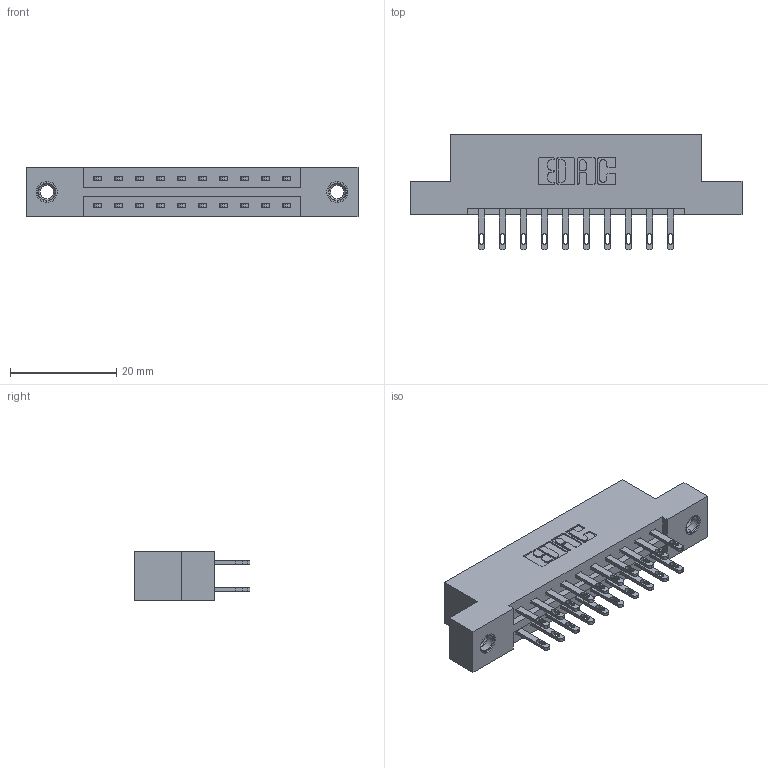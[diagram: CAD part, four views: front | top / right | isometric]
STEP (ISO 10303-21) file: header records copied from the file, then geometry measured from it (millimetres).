
FILE_DESCRIPTION (( 'STEP AP203' ), '1' );
FILE_NAME ('887-020-500-207.STEP', '2020-09-20T18:08:59', ( '' ), ( '' ), 'SwSTEP 2.0', 'SolidWorks 2020', '' );
FILE_SCHEMA (( 'CONFIG_CONTROL_DESIGN' ));
Length unit declared in the file: inch
Products named in the file (4): 345-292-001_345-293-100; 887-020-500-207; 837 Part_Flush Mounting Lugs - 0.156 Dia-TI; 345-250-001_345-250-005-103
Assembly tree (23 placements, depth 2):
  887-020-500-207
    837 Part_Flush Mounting Lugs - 0.156 Dia-TI
    345-292-001_345-293-100  x20
    345-250-001_345-250-005-103  x2
Bounding box: 62.64 x 21.85 x 9.4 mm (x, y, z)
Volume: 6222.8 mm3; surface area: 6981.9 mm2
Topology: 23 solids, 23 shells, 1174 faces, 3507 edges, 2330 vertices
Faces by surface type: plane 742, cylinder 416, cone 12, torus 4
Entity records: 13008 total; most frequent: CARTESIAN_POINT 2197, ORIENTED_EDGE 2126, DIRECTION 1961, EDGE_CURVE 1063, VECTOR 911, LINE 911, VERTEX_POINT 704, AXIS2_PLACEMENT_3D 525
